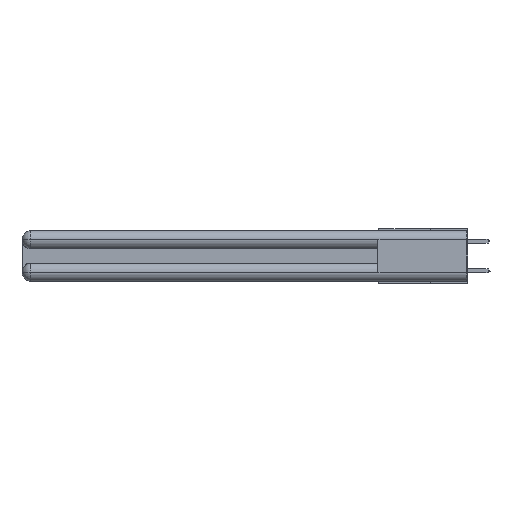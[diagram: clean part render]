
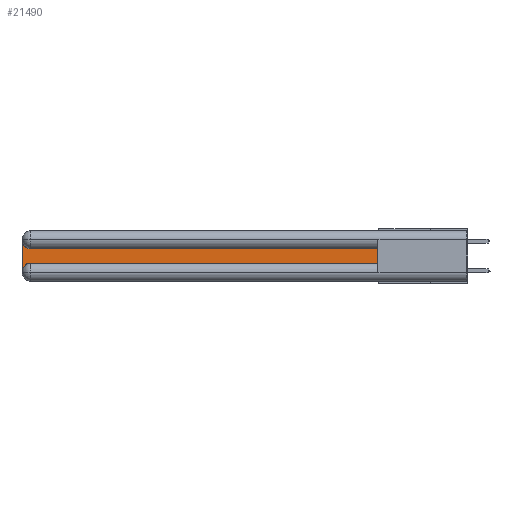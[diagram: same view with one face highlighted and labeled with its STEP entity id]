
A CAD part, left-side view. The second image highlights one B-rep face of the part: STEP entity #21490.
In plain terms, the highlighted planar face has unit normal (-1, 0, 0).
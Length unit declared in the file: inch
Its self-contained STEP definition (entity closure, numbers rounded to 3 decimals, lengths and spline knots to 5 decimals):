
#508 = ORIENTED_EDGE ( 'NONE', *, *, #12246, .T. ) ;
#1069 = DIRECTION ( 'NONE',  ( 0., -1., 0. ) ) ;
#1741 = FACE_OUTER_BOUND ( 'NONE', #18687, .T. ) ;
#2701 = EDGE_CURVE ( 'NONE', #32032, #29621, #30767, .T. ) ;
#3504 = ORIENTED_EDGE ( 'NONE', *, *, #34790, .T. ) ;
#3679 = VECTOR ( 'NONE', #28400, 39.37008 ) ;
#4077 = CARTESIAN_POINT ( 'NONE',  ( 0.075, 2.94, -0.0625 ) ) ;
#4079 = CARTESIAN_POINT ( 'NONE',  ( 0.075, 0.6, -0.1225 ) ) ;
#4695 = CIRCLE ( 'NONE', #28699, 0.06 ) ;
#4738 = EDGE_CURVE ( 'NONE', #24911, #32179, #29559, .T. ) ;
#6866 = DIRECTION ( 'NONE',  ( 0., 0., -1. ) ) ;
#7160 = CARTESIAN_POINT ( 'NONE',  ( 0.075, 2.94, -0.2775 ) ) ;
#7791 = CARTESIAN_POINT ( 'NONE',  ( 0.075, 3., -0.2175 ) ) ;
#8862 = CARTESIAN_POINT ( 'NONE',  ( 0.075, 0.6, -0.2175 ) ) ;
#9743 = LINE ( 'NONE', #4079, #3679 ) ;
#10611 = ORIENTED_EDGE ( 'NONE', *, *, #4738, .T. ) ;
#10774 = LINE ( 'NONE', #11778, #11193 ) ;
#11193 = VECTOR ( 'NONE', #1069, 39.37008 ) ;
#11778 = CARTESIAN_POINT ( 'NONE',  ( 0.075, 0.6, -0.2175 ) ) ;
#12246 = EDGE_CURVE ( 'NONE', #23148, #32032, #4695, .T. ) ;
#13705 = CARTESIAN_POINT ( 'NONE',  ( 0.075, 3., -0.2775 ) ) ;
#14455 = AXIS2_PLACEMENT_3D ( 'NONE', #7160, #28555, #17482 ) ;
#14606 = DIRECTION ( 'NONE',  ( 0., 0., -1. ) ) ;
#14739 = PLANE ( 'NONE',  #30550 ) ;
#14811 = CARTESIAN_POINT ( 'NONE',  ( 0.075, 2.94, -0.2175 ) ) ;
#15896 = CARTESIAN_POINT ( 'NONE',  ( 0.075, 3., -0.0625 ) ) ;
#15957 = DIRECTION ( 'NONE',  ( 0., 0., -1. ) ) ;
#17482 = DIRECTION ( 'NONE',  ( 0., 0., -1. ) ) ;
#18687 = EDGE_LOOP ( 'NONE', ( #19626, #508, #24499, #31938, #3504, #10611 ) ) ;
#19626 = ORIENTED_EDGE ( 'NONE', *, *, #31189, .T. ) ;
#19685 = DIRECTION ( 'NONE',  ( 0., 0., 1. ) ) ;
#21490 = ADVANCED_FACE ( 'NONE', ( #1741 ), #14739, .F. ) ;
#21726 = VECTOR ( 'NONE', #19685, 39.37008 ) ;
#23148 = VERTEX_POINT ( 'NONE', #29949 ) ;
#23184 = CARTESIAN_POINT ( 'NONE',  ( 0.075, 3., -0.1225 ) ) ;
#23409 = DIRECTION ( 'NONE',  ( 1., 0., 0. ) ) ;
#24499 = ORIENTED_EDGE ( 'NONE', *, *, #2701, .T. ) ;
#24911 = VERTEX_POINT ( 'NONE', #30072 ) ;
#27801 = CARTESIAN_POINT ( 'NONE',  ( 0.075, 0.6, -0.1225 ) ) ;
#28121 = VECTOR ( 'NONE', #15957, 39.37008 ) ;
#28400 = DIRECTION ( 'NONE',  ( 0., 1., 0. ) ) ;
#28555 = DIRECTION ( 'NONE',  ( 1., 0., 0. ) ) ;
#28699 = AXIS2_PLACEMENT_3D ( 'NONE', #4077, #23409, #6866 ) ;
#29559 = LINE ( 'NONE', #8862, #21726 ) ;
#29621 = VERTEX_POINT ( 'NONE', #13705 ) ;
#29949 = CARTESIAN_POINT ( 'NONE',  ( 0.075, 2.94, -0.1225 ) ) ;
#30072 = CARTESIAN_POINT ( 'NONE',  ( 0.075, 0.6, -0.2175 ) ) ;
#30550 = AXIS2_PLACEMENT_3D ( 'NONE', #23184, #33933, #14606 ) ;
#30767 = LINE ( 'NONE', #7791, #28121 ) ;
#30992 = CIRCLE ( 'NONE', #14455, 0.06 ) ;
#31189 = EDGE_CURVE ( 'NONE', #32179, #23148, #9743, .T. ) ;
#31310 = EDGE_CURVE ( 'NONE', #29621, #35128, #30992, .T. ) ;
#31938 = ORIENTED_EDGE ( 'NONE', *, *, #31310, .T. ) ;
#32032 = VERTEX_POINT ( 'NONE', #15896 ) ;
#32179 = VERTEX_POINT ( 'NONE', #27801 ) ;
#33933 = DIRECTION ( 'NONE',  ( 1., 0., 0. ) ) ;
#34790 = EDGE_CURVE ( 'NONE', #35128, #24911, #10774, .T. ) ;
#35128 = VERTEX_POINT ( 'NONE', #14811 ) ;
